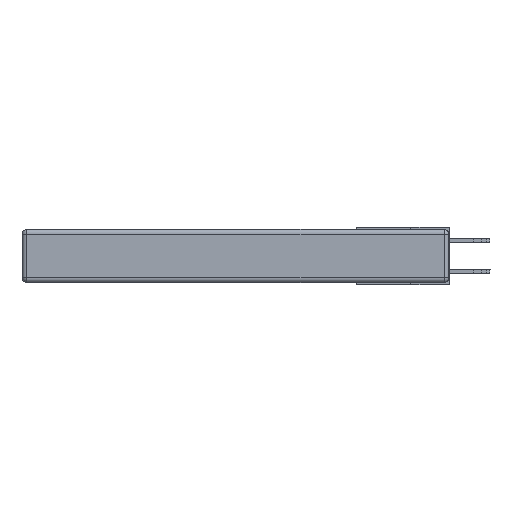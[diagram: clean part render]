
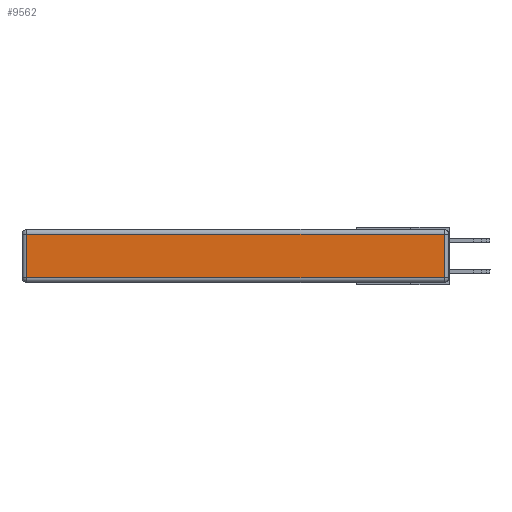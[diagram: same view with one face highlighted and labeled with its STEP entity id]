
A CAD part, left-side view. The second image highlights one B-rep face of the part: STEP entity #9562.
In plain terms, the highlighted planar face has unit normal (-1, 0, 0).
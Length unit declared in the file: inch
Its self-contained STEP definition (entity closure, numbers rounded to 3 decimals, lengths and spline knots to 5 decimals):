
#122 = VECTOR ( 'NONE', #15668, 39.37008 ) ;
#270 = CARTESIAN_POINT ( 'NONE',  ( 0., 0.03, -0.313 ) ) ;
#757 = ORIENTED_EDGE ( 'NONE', *, *, #9051, .T. ) ;
#798 = FACE_OUTER_BOUND ( 'NONE', #9594, .T. ) ;
#870 = VERTEX_POINT ( 'NONE', #270 ) ;
#1002 = VECTOR ( 'NONE', #17938, 39.37008 ) ;
#1010 = VERTEX_POINT ( 'NONE', #7546 ) ;
#1576 = LINE ( 'NONE', #2804, #11368 ) ;
#1880 = VERTEX_POINT ( 'NONE', #3087 ) ;
#2291 = CARTESIAN_POINT ( 'NONE',  ( 0., 2.75, -0.03 ) ) ;
#2598 = LINE ( 'NONE', #9955, #122 ) ;
#2804 = CARTESIAN_POINT ( 'NONE',  ( 0., 0., -0.313 ) ) ;
#3087 = CARTESIAN_POINT ( 'NONE',  ( 0., 2.72, -0.313 ) ) ;
#3745 = PLANE ( 'NONE',  #10937 ) ;
#6588 = CARTESIAN_POINT ( 'NONE',  ( 0., 0., -0.343 ) ) ;
#7054 = LINE ( 'NONE', #16904, #9264 ) ;
#7546 = CARTESIAN_POINT ( 'NONE',  ( 0., 2.72, -0.03 ) ) ;
#7596 = VERTEX_POINT ( 'NONE', #13277 ) ;
#8060 = DIRECTION ( 'NONE',  ( -1., 0., 0. ) ) ;
#9051 = EDGE_CURVE ( 'NONE', #870, #7596, #2598, .T. ) ;
#9179 = EDGE_CURVE ( 'NONE', #1010, #1880, #7054, .T. ) ;
#9264 = VECTOR ( 'NONE', #14291, 39.37008 ) ;
#9492 = DIRECTION ( 'NONE',  ( 0., 0., 1. ) ) ;
#9562 = ADVANCED_FACE ( 'NONE', ( #798 ), #3745, .T. ) ;
#9594 = EDGE_LOOP ( 'NONE', ( #12454, #757, #9852, #10677 ) ) ;
#9695 = DIRECTION ( 'NONE',  ( 0., -1., 0. ) ) ;
#9852 = ORIENTED_EDGE ( 'NONE', *, *, #14860, .T. ) ;
#9955 = CARTESIAN_POINT ( 'NONE',  ( 0., 0.03, -0.343 ) ) ;
#10677 = ORIENTED_EDGE ( 'NONE', *, *, #9179, .T. ) ;
#10937 = AXIS2_PLACEMENT_3D ( 'NONE', #6588, #8060, #9492 ) ;
#11368 = VECTOR ( 'NONE', #9695, 39.37008 ) ;
#11698 = LINE ( 'NONE', #2291, #1002 ) ;
#12454 = ORIENTED_EDGE ( 'NONE', *, *, #16884, .T. ) ;
#13277 = CARTESIAN_POINT ( 'NONE',  ( 0., 0.03, -0.03 ) ) ;
#14291 = DIRECTION ( 'NONE',  ( 0., 0., -1. ) ) ;
#14860 = EDGE_CURVE ( 'NONE', #7596, #1010, #11698, .T. ) ;
#15668 = DIRECTION ( 'NONE',  ( 0., 0., 1. ) ) ;
#16884 = EDGE_CURVE ( 'NONE', #1880, #870, #1576, .T. ) ;
#16904 = CARTESIAN_POINT ( 'NONE',  ( 0., 2.72, -0.343 ) ) ;
#17938 = DIRECTION ( 'NONE',  ( 0., 1., 0. ) ) ;
